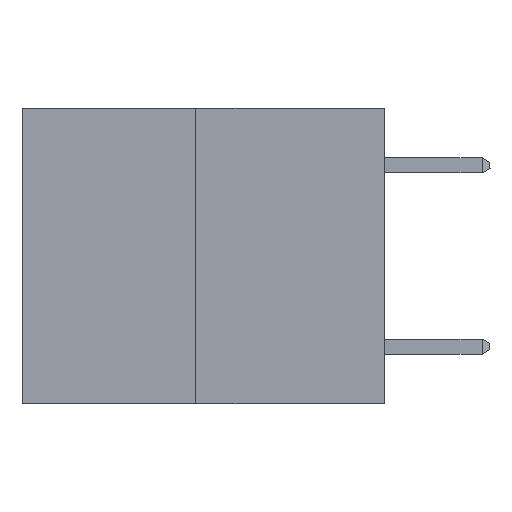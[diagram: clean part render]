
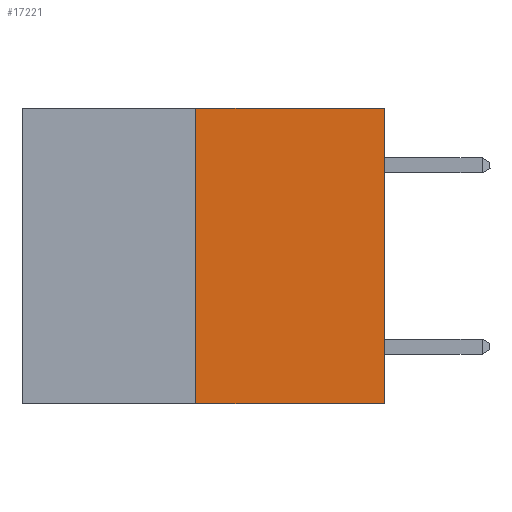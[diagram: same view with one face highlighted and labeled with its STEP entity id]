
A CAD part, left-side view. The second image highlights one B-rep face of the part: STEP entity #17221.
In plain terms, the highlighted planar face has unit normal (-1, 0, 0).
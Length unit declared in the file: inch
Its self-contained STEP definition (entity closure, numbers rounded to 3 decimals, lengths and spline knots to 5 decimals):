
#661 = VECTOR ( 'NONE', #21122, 39.37008 ) ;
#2939 = LINE ( 'NONE', #23138, #27498 ) ;
#3429 = EDGE_CURVE ( 'NONE', #6308, #14998, #23606, .T. ) ;
#4384 = VECTOR ( 'NONE', #27846, 39.37008 ) ;
#5703 = EDGE_LOOP ( 'NONE', ( #9073, #13732, #7751, #19379 ) ) ;
#5742 = DIRECTION ( 'NONE',  ( 0., 0., 1. ) ) ;
#5745 = LINE ( 'NONE', #23468, #4384 ) ;
#5766 = AXIS2_PLACEMENT_3D ( 'NONE', #26926, #20419, #16052 ) ;
#6157 = FACE_OUTER_BOUND ( 'NONE', #5703, .T. ) ;
#6308 = VERTEX_POINT ( 'NONE', #6752 ) ;
#6752 = CARTESIAN_POINT ( 'NONE',  ( 0., 0.312, -0.49 ) ) ;
#7751 = ORIENTED_EDGE ( 'NONE', *, *, #20612, .T. ) ;
#9073 = ORIENTED_EDGE ( 'NONE', *, *, #3429, .F. ) ;
#10582 = VERTEX_POINT ( 'NONE', #13727 ) ;
#10712 = VERTEX_POINT ( 'NONE', #18656 ) ;
#10739 = EDGE_CURVE ( 'NONE', #6308, #10712, #25230, .T. ) ;
#11499 = PLANE ( 'NONE',  #5766 ) ;
#12232 = CARTESIAN_POINT ( 'NONE',  ( 0., 0.312, -0.49 ) ) ;
#12287 = DIRECTION ( 'NONE',  ( 0., -1., 0. ) ) ;
#12961 = CARTESIAN_POINT ( 'NONE',  ( 0., 0.312, 0. ) ) ;
#13727 = CARTESIAN_POINT ( 'NONE',  ( 0., 0., 0. ) ) ;
#13732 = ORIENTED_EDGE ( 'NONE', *, *, #10739, .T. ) ;
#14998 = VERTEX_POINT ( 'NONE', #12961 ) ;
#16052 = DIRECTION ( 'NONE',  ( 0., 0., -1. ) ) ;
#16119 = VECTOR ( 'NONE', #5742, 39.37008 ) ;
#17221 = ADVANCED_FACE ( 'NONE', ( #6157 ), #11499, .F. ) ;
#18656 = CARTESIAN_POINT ( 'NONE',  ( 0., 0., -0.49 ) ) ;
#19379 = ORIENTED_EDGE ( 'NONE', *, *, #22589, .F. ) ;
#20419 = DIRECTION ( 'NONE',  ( 1., 0., 0. ) ) ;
#20612 = EDGE_CURVE ( 'NONE', #10712, #10582, #5745, .T. ) ;
#21122 = DIRECTION ( 'NONE',  ( 0., -1., 0. ) ) ;
#22589 = EDGE_CURVE ( 'NONE', #14998, #10582, #2939, .T. ) ;
#23138 = CARTESIAN_POINT ( 'NONE',  ( 0., 0.6, 0. ) ) ;
#23334 = CARTESIAN_POINT ( 'NONE',  ( 0., 0.6, -0.49 ) ) ;
#23468 = CARTESIAN_POINT ( 'NONE',  ( 0., 0., 0. ) ) ;
#23606 = LINE ( 'NONE', #12232, #16119 ) ;
#25230 = LINE ( 'NONE', #23334, #661 ) ;
#26926 = CARTESIAN_POINT ( 'NONE',  ( 0., 0.6, 0. ) ) ;
#27498 = VECTOR ( 'NONE', #12287, 39.37008 ) ;
#27846 = DIRECTION ( 'NONE',  ( 0., 0., 1. ) ) ;
